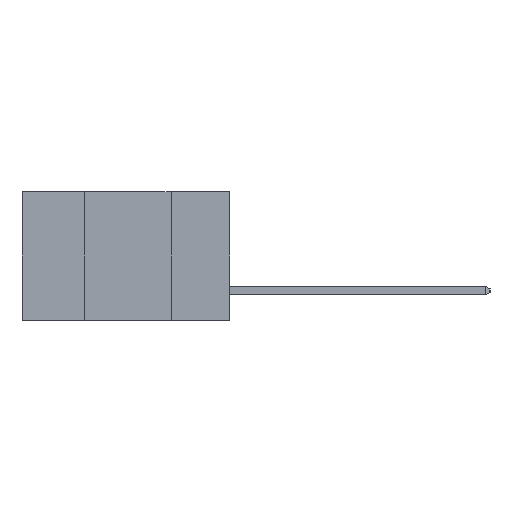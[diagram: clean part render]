
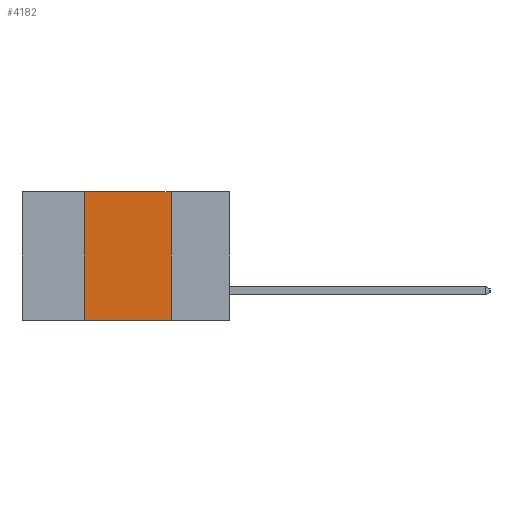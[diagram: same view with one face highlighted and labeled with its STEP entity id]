
A CAD part, left-side view. The second image highlights one B-rep face of the part: STEP entity #4182.
In plain terms, the highlighted planar face has unit normal (-1, 0, 0).
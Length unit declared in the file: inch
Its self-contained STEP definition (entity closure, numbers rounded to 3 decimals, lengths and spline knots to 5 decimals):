
#511 = LINE ( 'NONE', #7989, #15001 ) ;
#1037 = AXIS2_PLACEMENT_3D ( 'NONE', #9547, #2470, #2618 ) ;
#1696 = VERTEX_POINT ( 'NONE', #2878 ) ;
#2088 = FACE_OUTER_BOUND ( 'NONE', #9834, .T. ) ;
#2383 = VECTOR ( 'NONE', #12263, 39.37008 ) ;
#2470 = DIRECTION ( 'NONE',  ( 1., 0., 0. ) ) ;
#2505 = VERTEX_POINT ( 'NONE', #15164 ) ;
#2618 = DIRECTION ( 'NONE',  ( 0., 0., -1. ) ) ;
#2878 = CARTESIAN_POINT ( 'NONE',  ( 0., 0.42, 0. ) ) ;
#3163 = EDGE_CURVE ( 'NONE', #10583, #2505, #13942, .T. ) ;
#3512 = DIRECTION ( 'NONE',  ( 0., 0., -1. ) ) ;
#3736 = EDGE_CURVE ( 'NONE', #1696, #17649, #511, .T. ) ;
#4182 = ADVANCED_FACE ( 'NONE', ( #2088 ), #15841, .F. ) ;
#6104 = EDGE_CURVE ( 'NONE', #10583, #1696, #6640, .T. ) ;
#6416 = DIRECTION ( 'NONE',  ( 0., -1., 0. ) ) ;
#6462 = CARTESIAN_POINT ( 'NONE',  ( 0., 0.6, -0.37 ) ) ;
#6640 = LINE ( 'NONE', #16774, #17406 ) ;
#7989 = CARTESIAN_POINT ( 'NONE',  ( 0., 0.6, 0. ) ) ;
#8671 = LINE ( 'NONE', #12155, #16156 ) ;
#9037 = CARTESIAN_POINT ( 'NONE',  ( 0., 0.17, 0. ) ) ;
#9162 = CARTESIAN_POINT ( 'NONE',  ( 0., 0.42, -0.37 ) ) ;
#9547 = CARTESIAN_POINT ( 'NONE',  ( 0., 0.6, 0. ) ) ;
#9834 = EDGE_LOOP ( 'NONE', ( #12294, #18194, #13806, #17714 ) ) ;
#10583 = VERTEX_POINT ( 'NONE', #9162 ) ;
#12155 = CARTESIAN_POINT ( 'NONE',  ( 0., 0.17, 0. ) ) ;
#12263 = DIRECTION ( 'NONE',  ( 0., -1., 0. ) ) ;
#12294 = ORIENTED_EDGE ( 'NONE', *, *, #13821, .F. ) ;
#13806 = ORIENTED_EDGE ( 'NONE', *, *, #6104, .F. ) ;
#13821 = EDGE_CURVE ( 'NONE', #17649, #2505, #8671, .T. ) ;
#13942 = LINE ( 'NONE', #6462, #2383 ) ;
#15001 = VECTOR ( 'NONE', #6416, 39.37008 ) ;
#15164 = CARTESIAN_POINT ( 'NONE',  ( 0., 0.17, -0.37 ) ) ;
#15841 = PLANE ( 'NONE',  #1037 ) ;
#16156 = VECTOR ( 'NONE', #3512, 39.37008 ) ;
#16660 = DIRECTION ( 'NONE',  ( 0., 0., 1. ) ) ;
#16774 = CARTESIAN_POINT ( 'NONE',  ( 0., 0.42, 0. ) ) ;
#17406 = VECTOR ( 'NONE', #16660, 39.37008 ) ;
#17649 = VERTEX_POINT ( 'NONE', #9037 ) ;
#17714 = ORIENTED_EDGE ( 'NONE', *, *, #3163, .T. ) ;
#18194 = ORIENTED_EDGE ( 'NONE', *, *, #3736, .F. ) ;
